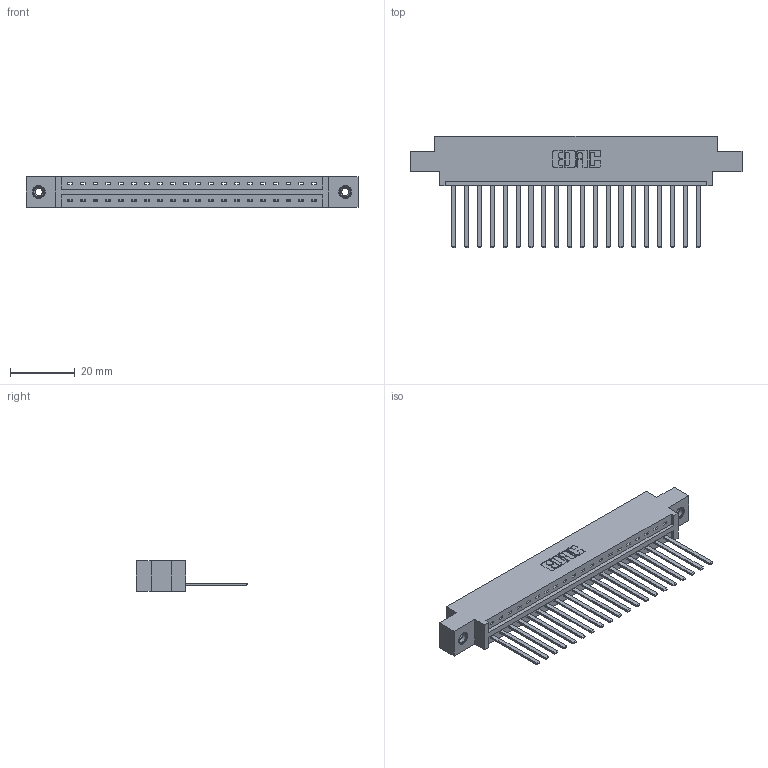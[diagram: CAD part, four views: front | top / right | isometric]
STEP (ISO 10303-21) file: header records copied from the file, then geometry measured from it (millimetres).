
FILE_DESCRIPTION (( 'STEP AP203' ), '1' );
FILE_NAME ('387-020-544-608.STEP', '2018-09-13T11:52:45', ( '' ), ( '' ), 'SwSTEP 2.0', 'SolidWorks 2016', '' );
FILE_SCHEMA (( 'CONFIG_CONTROL_DESIGN' ));
Length unit declared in the file: inch
Products named in the file (4): 345-292-001_345-293-144; 345-250-001_345-250-003-102; 387-020-544-608; 337 Part_0.170 Offset - 0.156 Dia-TI
Assembly tree (23 placements, depth 2):
  387-020-544-608
    337 Part_0.170 Offset - 0.156 Dia-TI
    345-292-001_345-293-144  x20
    345-250-001_345-250-003-102  x2
Bounding box: 102.26 x 34.3 x 9.4 mm (x, y, z)
Volume: 10460.5 mm3; surface area: 11575.4 mm2
Topology: 23 solids, 23 shells, 1298 faces, 3859 edges, 2538 vertices
Faces by surface type: plane 946, cylinder 336, cone 12, torus 4
Entity records: 18846 total; most frequent: CARTESIAN_POINT 3261, ORIENTED_EDGE 3210, DIRECTION 2819, EDGE_CURVE 1605, LINE 1461, VECTOR 1461, VERTEX_POINT 1064, AXIS2_PLACEMENT_3D 679
